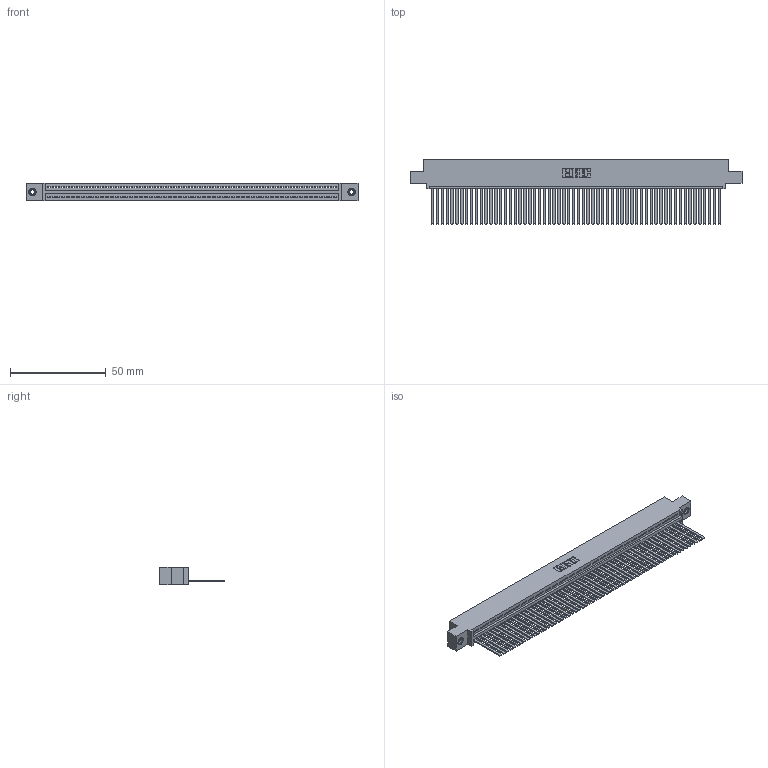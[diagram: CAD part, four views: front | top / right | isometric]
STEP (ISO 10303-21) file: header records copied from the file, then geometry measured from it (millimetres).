
FILE_DESCRIPTION (( 'STEP AP203' ), '1' );
FILE_NAME ('345-060-544-408.STEP', '2018-09-27T03:15:33', ( '' ), ( '' ), 'SwSTEP 2.0', 'SolidWorks 2016', '' );
FILE_SCHEMA (( 'CONFIG_CONTROL_DESIGN' ));
Length unit declared in the file: inch
Products named in the file (4): 345-060-544-408; 345-250-001_345-250-003-102; 345 Part_0.110 Offset - 0.156 Dia-TI; 345-292-001_345-293-144
Assembly tree (63 placements, depth 2):
  345-060-544-408
    345 Part_0.110 Offset - 0.156 Dia-TI
    345-292-001_345-293-144  x60
    345-250-001_345-250-003-102  x2
Bounding box: 173.61 x 33.96 x 9.4 mm (x, y, z)
Volume: 17252 mm3; surface area: 25358.1 mm2
Topology: 63 solids, 63 shells, 3310 faces, 9969 edges, 6558 vertices
Faces by surface type: plane 2276, cylinder 1018, cone 12, torus 4
Entity records: 43868 total; most frequent: CARTESIAN_POINT 7579, ORIENTED_EDGE 7566, DIRECTION 6617, EDGE_CURVE 3783, LINE 3395, VECTOR 3395, VERTEX_POINT 2516, AXIS2_PLACEMENT_3D 1611
